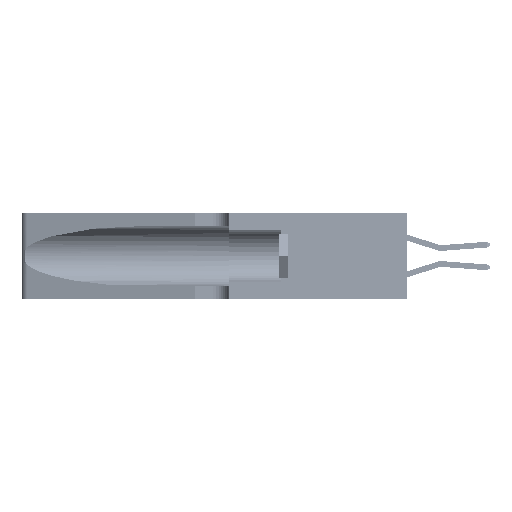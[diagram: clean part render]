
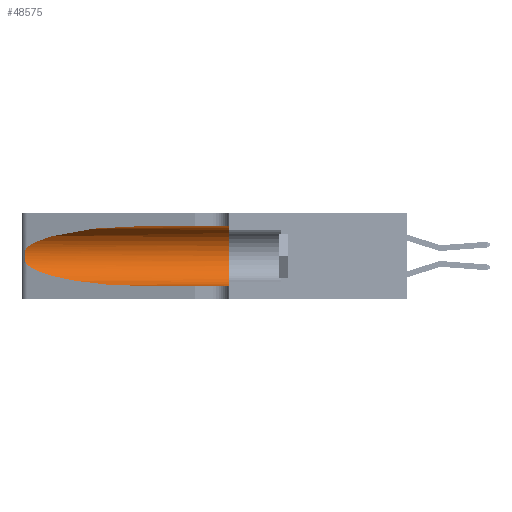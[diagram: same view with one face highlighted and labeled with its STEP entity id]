
A CAD part, left-side view. The second image highlights one B-rep face of the part: STEP entity #48575.
In plain terms, the highlighted cylindrical face has radius 3.308 mm (diameter 6.617 mm), a partial arc.
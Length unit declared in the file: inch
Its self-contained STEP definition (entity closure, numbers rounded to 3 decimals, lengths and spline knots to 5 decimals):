
#80 = CARTESIAN_POINT ( 'NONE',  ( 0.2373, 1.15595, 0.08982 ) ) ;
#628 = EDGE_CURVE ( 'NONE', #21006, #33146, #31721, .T. ) ;
#1172 = CARTESIAN_POINT ( 'NONE',  ( 0.25487, 1.22718, 0.14631 ) ) ;
#1698 = EDGE_CURVE ( 'NONE', #30555, #42501, #5396, .T. ) ;
#2454 = CIRCLE ( 'NONE', #30257, 0.13025 ) ;
#2531 = FACE_OUTER_BOUND ( 'NONE', #42709, .T. ) ;
#3934 = CARTESIAN_POINT ( 'NONE',  ( 0.25487, 1.22718, 0.14631 ) ) ;
#4554 = VECTOR ( 'NONE', #29573, 39.37008 ) ;
#5396 =( BOUNDED_CURVE ( )  B_SPLINE_CURVE ( 3, ( #34693, #23429, #34365, #8264 ),
 .UNSPECIFIED., .F., .F. ) 
 B_SPLINE_CURVE_WITH_KNOTS ( ( 4, 4 ),
 ( 1.5708, 2.84003 ),
 .UNSPECIFIED. ) 
 CURVE ( )  GEOMETRIC_REPRESENTATION_ITEM ( )  RATIONAL_B_SPLINE_CURVE ( ( 1., 0.87, 0.87, 1. ) ) 
 REPRESENTATION_ITEM ( '' )  );
#6128 = ORIENTED_EDGE ( 'NONE', *, *, #14233, .T. ) ;
#6473 = CARTESIAN_POINT ( 'NONE',  ( 0.25487, 1.22718, 0.22369 ) ) ;
#6830 = CARTESIAN_POINT ( 'NONE',  ( 0.1305, 0.35, 0.185 ) ) ;
#7218 = CARTESIAN_POINT ( 'NONE',  ( 0.25639, 1.23186, 0.15144 ) ) ;
#7381 = CARTESIAN_POINT ( 'NONE',  ( 0.25555, 1.22994, 0.2215 ) ) ;
#8264 = CARTESIAN_POINT ( 'NONE',  ( 0.25487, 1.22718, 0.22369 ) ) ;
#9260 = ORIENTED_EDGE ( 'NONE', *, *, #17787, .T. ) ;
#10168 = DIRECTION ( 'NONE',  ( 0., -1., 0. ) ) ;
#11163 = CARTESIAN_POINT ( 'NONE',  ( 0.25854, 1.2359, 0.20912 ) ) ;
#11326 = CARTESIAN_POINT ( 'NONE',  ( 0.25487, 1.22718, 0.22369 ) ) ;
#11467 = LINE ( 'NONE', #22036, #38115 ) ;
#11498 = CARTESIAN_POINT ( 'NONE',  ( 0.25787, 1.23484, 0.2124 ) ) ;
#12812 = EDGE_CURVE ( 'NONE', #30555, #44897, #11467, .T. ) ;
#14233 = EDGE_CURVE ( 'NONE', #42501, #21006, #36898, .T. ) ;
#15073 = ORIENTED_EDGE ( 'NONE', *, *, #628, .T. ) ;
#15074 = CARTESIAN_POINT ( 'NONE',  ( 0.18966, 0.96281, 0.05475 ) ) ;
#17787 = EDGE_CURVE ( 'NONE', #33146, #42562, #18677, .T. ) ;
#18037 = CARTESIAN_POINT ( 'NONE',  ( 0.1305, 1.61858, 0.05475 ) ) ;
#18410 = DIRECTION ( 'NONE',  ( 0., 0., -1. ) ) ;
#18677 = LINE ( 'NONE', #18037, #4554 ) ;
#21006 = VERTEX_POINT ( 'NONE', #1172 ) ;
#21951 = CYLINDRICAL_SURFACE ( 'NONE', #41626, 0.13025 ) ;
#22036 = CARTESIAN_POINT ( 'NONE',  ( 0.1305, 1.61858, 0.31525 ) ) ;
#22870 = CARTESIAN_POINT ( 'NONE',  ( 0.26018, 1.23835, 0.19895 ) ) ;
#23429 = CARTESIAN_POINT ( 'NONE',  ( 0.18966, 0.96281, 0.31525 ) ) ;
#26200 = CARTESIAN_POINT ( 'NONE',  ( 0.26075, 1.23896, 0.178 ) ) ;
#28027 = CARTESIAN_POINT ( 'NONE',  ( 0.1305, 0.35, 0.31525 ) ) ;
#28056 = EDGE_CURVE ( 'NONE', #44897, #42562, #2454, .T. ) ;
#29573 = DIRECTION ( 'NONE',  ( 0., -1., 0. ) ) ;
#29818 = CARTESIAN_POINT ( 'NONE',  ( 0.1305, 0.72297, 0.05475 ) ) ;
#30240 = CARTESIAN_POINT ( 'NONE',  ( 0.1305, 0.72297, 0.05475 ) ) ;
#30257 = AXIS2_PLACEMENT_3D ( 'NONE', #6830, #33250, #40270 ) ;
#30461 = CARTESIAN_POINT ( 'NONE',  ( 0.25639, 1.23184, 0.21858 ) ) ;
#30555 = VERTEX_POINT ( 'NONE', #47797 ) ;
#31246 = ORIENTED_EDGE ( 'NONE', *, *, #12812, .F. ) ;
#31721 =( BOUNDED_CURVE ( )  B_SPLINE_CURVE ( 3, ( #33927, #80, #15074, #30240 ),
 .UNSPECIFIED., .F., .F. ) 
 B_SPLINE_CURVE_WITH_KNOTS ( ( 4, 4 ),
 ( 3.44316, 4.71239 ),
 .UNSPECIFIED. ) 
 CURVE ( )  GEOMETRIC_REPRESENTATION_ITEM ( )  RATIONAL_B_SPLINE_CURVE ( ( 1., 0.87, 0.87, 1. ) ) 
 REPRESENTATION_ITEM ( '' )  );
#33146 = VERTEX_POINT ( 'NONE', #29818 ) ;
#33250 = DIRECTION ( 'NONE',  ( 0., 1., 0. ) ) ;
#33801 = CARTESIAN_POINT ( 'NONE',  ( 0.26017, 1.23833, 0.17102 ) ) ;
#33927 = CARTESIAN_POINT ( 'NONE',  ( 0.25487, 1.22718, 0.14631 ) ) ;
#34365 = CARTESIAN_POINT ( 'NONE',  ( 0.2373, 1.15595, 0.28018 ) ) ;
#34693 = CARTESIAN_POINT ( 'NONE',  ( 0.1305, 0.72297, 0.31525 ) ) ;
#36898 = B_SPLINE_CURVE_WITH_KNOTS ( 'NONE', 3,
 ( #11326, #7381, #30461, #11498, #11163, #22870, #48962, #26200, #33801, #41639, #41814, #7218, #38140, #3934 ),
 .UNSPECIFIED., .F., .F.,
 ( 4, 2, 2, 2, 2, 2, 4 ),
 ( 0., 0.00027, 0.00053, 0.00107, 0.0016, 0.00187, 0.00214 ),
 .UNSPECIFIED. ) ;
#38115 = VECTOR ( 'NONE', #10168, 39.37008 ) ;
#38140 = CARTESIAN_POINT ( 'NONE',  ( 0.25555, 1.22993, 0.14849 ) ) ;
#39285 = ORIENTED_EDGE ( 'NONE', *, *, #1698, .T. ) ;
#40270 = DIRECTION ( 'NONE',  ( 0., 0., 1. ) ) ;
#41298 = CARTESIAN_POINT ( 'NONE',  ( 0.1305, 1.61858, 0.185 ) ) ;
#41540 = CARTESIAN_POINT ( 'NONE',  ( 0.1305, 0.35, 0.05475 ) ) ;
#41626 = AXIS2_PLACEMENT_3D ( 'NONE', #41298, #48625, #18410 ) ;
#41639 = CARTESIAN_POINT ( 'NONE',  ( 0.25856, 1.23593, 0.16098 ) ) ;
#41814 = CARTESIAN_POINT ( 'NONE',  ( 0.25789, 1.23486, 0.15765 ) ) ;
#42501 = VERTEX_POINT ( 'NONE', #6473 ) ;
#42562 = VERTEX_POINT ( 'NONE', #41540 ) ;
#42709 = EDGE_LOOP ( 'NONE', ( #39285, #6128, #15073, #9260, #47989, #31246 ) ) ;
#44897 = VERTEX_POINT ( 'NONE', #28027 ) ;
#47797 = CARTESIAN_POINT ( 'NONE',  ( 0.1305, 0.72297, 0.31525 ) ) ;
#47989 = ORIENTED_EDGE ( 'NONE', *, *, #28056, .F. ) ;
#48575 = ADVANCED_FACE ( 'NONE', ( #2531 ), #21951, .F. ) ;
#48625 = DIRECTION ( 'NONE',  ( 0., -1., 0. ) ) ;
#48962 = CARTESIAN_POINT ( 'NONE',  ( 0.26075, 1.23896, 0.19203 ) ) ;
